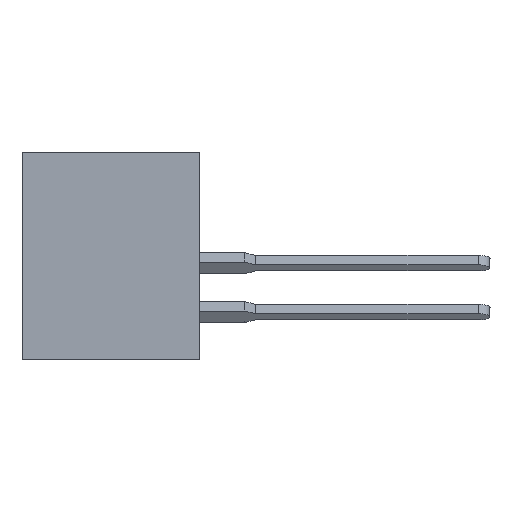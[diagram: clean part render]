
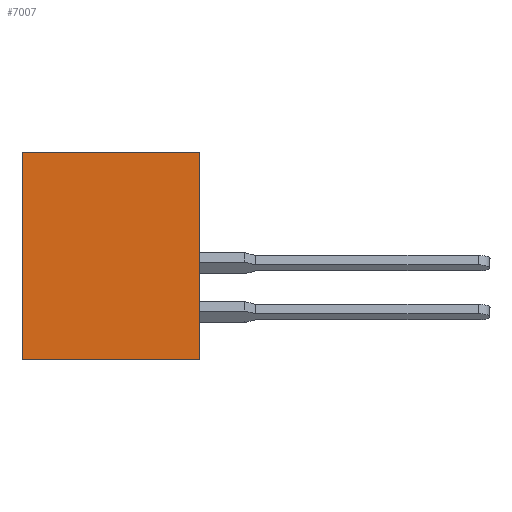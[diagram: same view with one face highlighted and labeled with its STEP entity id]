
A CAD part, left-side view. The second image highlights one B-rep face of the part: STEP entity #7007.
In plain terms, the highlighted planar face has unit normal (-1, 0, 0).
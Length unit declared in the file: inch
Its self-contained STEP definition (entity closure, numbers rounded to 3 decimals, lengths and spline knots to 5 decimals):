
#437 = ORIENTED_EDGE ( 'NONE', *, *, #5606, .T. ) ;
#839 = AXIS2_PLACEMENT_3D ( 'NONE', #16563, #6013, #7692 ) ;
#968 = VERTEX_POINT ( 'NONE', #5648 ) ;
#1649 = PLANE ( 'NONE',  #839 ) ;
#1791 = EDGE_CURVE ( 'NONE', #10640, #18723, #3521, .T. ) ;
#2572 = LINE ( 'NONE', #4105, #14938 ) ;
#2946 = EDGE_CURVE ( 'NONE', #9680, #10640, #19290, .T. ) ;
#3360 = CARTESIAN_POINT ( 'NONE',  ( 0., 0.453, -0.531 ) ) ;
#3508 = CARTESIAN_POINT ( 'NONE',  ( 0., 0.453, 0. ) ) ;
#3521 = LINE ( 'NONE', #3508, #18413 ) ;
#4105 = CARTESIAN_POINT ( 'NONE',  ( 0., 0., 0. ) ) ;
#4349 = CARTESIAN_POINT ( 'NONE',  ( 0., 0.453, -0.531 ) ) ;
#5495 = DIRECTION ( 'NONE',  ( 0., 0., 1. ) ) ;
#5606 = EDGE_CURVE ( 'NONE', #968, #18723, #2572, .T. ) ;
#5648 = CARTESIAN_POINT ( 'NONE',  ( 0., 0., -0.531 ) ) ;
#6013 = DIRECTION ( 'NONE',  ( 1., 0., 0. ) ) ;
#6243 = EDGE_CURVE ( 'NONE', #9680, #968, #10680, .T. ) ;
#6996 = DIRECTION ( 'NONE',  ( 0., 0., 1. ) ) ;
#7007 = ADVANCED_FACE ( 'NONE', ( #13053 ), #1649, .F. ) ;
#7233 = DIRECTION ( 'NONE',  ( 0., -1., 0. ) ) ;
#7334 = ORIENTED_EDGE ( 'NONE', *, *, #2946, .F. ) ;
#7692 = DIRECTION ( 'NONE',  ( 0., 0., -1. ) ) ;
#8689 = ORIENTED_EDGE ( 'NONE', *, *, #1791, .F. ) ;
#9680 = VERTEX_POINT ( 'NONE', #3360 ) ;
#10640 = VERTEX_POINT ( 'NONE', #16859 ) ;
#10680 = LINE ( 'NONE', #4349, #16983 ) ;
#12279 = VECTOR ( 'NONE', #5495, 39.37008 ) ;
#12928 = CARTESIAN_POINT ( 'NONE',  ( 0., 0.453, 0. ) ) ;
#13053 = FACE_OUTER_BOUND ( 'NONE', #13054, .T. ) ;
#13054 = EDGE_LOOP ( 'NONE', ( #437, #8689, #7334, #13403 ) ) ;
#13403 = ORIENTED_EDGE ( 'NONE', *, *, #6243, .T. ) ;
#13781 = DIRECTION ( 'NONE',  ( 0., -1., 0. ) ) ;
#14523 = CARTESIAN_POINT ( 'NONE',  ( 0., 0., 0. ) ) ;
#14938 = VECTOR ( 'NONE', #6996, 39.37008 ) ;
#16563 = CARTESIAN_POINT ( 'NONE',  ( 0., 0.453, 0. ) ) ;
#16859 = CARTESIAN_POINT ( 'NONE',  ( 0., 0.453, 0. ) ) ;
#16983 = VECTOR ( 'NONE', #7233, 39.37008 ) ;
#18413 = VECTOR ( 'NONE', #13781, 39.37008 ) ;
#18723 = VERTEX_POINT ( 'NONE', #14523 ) ;
#19290 = LINE ( 'NONE', #12928, #12279 ) ;
